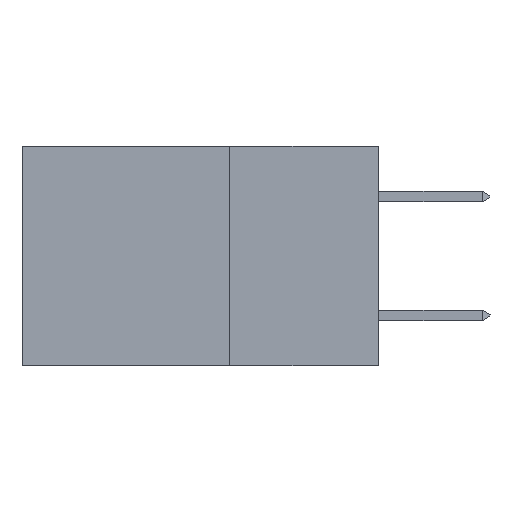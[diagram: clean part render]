
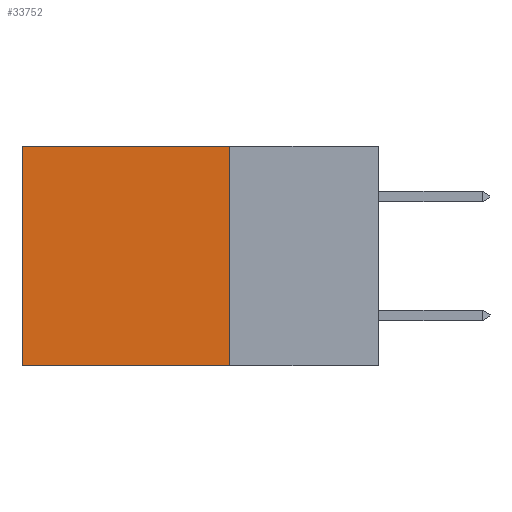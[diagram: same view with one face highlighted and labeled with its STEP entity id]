
A CAD part, left-side view. The second image highlights one B-rep face of the part: STEP entity #33752.
In plain terms, the highlighted planar face has unit normal (-1, 0, 0).
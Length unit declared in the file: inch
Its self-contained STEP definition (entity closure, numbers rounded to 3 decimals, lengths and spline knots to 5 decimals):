
#383 = LINE ( 'NONE', #13626, #21250 ) ;
#1991 = LINE ( 'NONE', #14796, #5744 ) ;
#3336 = VERTEX_POINT ( 'NONE', #23021 ) ;
#4294 = ORIENTED_EDGE ( 'NONE', *, *, #11219, .T. ) ;
#4408 = CARTESIAN_POINT ( 'NONE',  ( 0.298, 0.25, 0. ) ) ;
#4833 = FACE_OUTER_BOUND ( 'NONE', #34404, .T. ) ;
#5744 = VECTOR ( 'NONE', #24946, 39.37008 ) ;
#5864 = EDGE_CURVE ( 'NONE', #24823, #3336, #1991, .T. ) ;
#5874 = CARTESIAN_POINT ( 'NONE',  ( 0.298, 0.25, -0.37 ) ) ;
#6269 = LINE ( 'NONE', #25279, #28749 ) ;
#8579 = LINE ( 'NONE', #21059, #11482 ) ;
#10102 = DIRECTION ( 'NONE',  ( 1., 0., 0. ) ) ;
#10293 = VERTEX_POINT ( 'NONE', #10602 ) ;
#10329 = DIRECTION ( 'NONE',  ( 0., 0., -1. ) ) ;
#10602 = CARTESIAN_POINT ( 'NONE',  ( 0.298, 0.6, 0. ) ) ;
#11219 = EDGE_CURVE ( 'NONE', #10293, #3336, #8579, .T. ) ;
#11482 = VECTOR ( 'NONE', #34122, 39.37008 ) ;
#13626 = CARTESIAN_POINT ( 'NONE',  ( 0.298, 0.25, 0. ) ) ;
#14796 = CARTESIAN_POINT ( 'NONE',  ( 0.298, 0.25, -0.37 ) ) ;
#16840 = EDGE_CURVE ( 'NONE', #27444, #24823, #383, .T. ) ;
#17937 = DIRECTION ( 'NONE',  ( 0., 1., 0. ) ) ;
#20453 = ORIENTED_EDGE ( 'NONE', *, *, #5864, .F. ) ;
#21059 = CARTESIAN_POINT ( 'NONE',  ( 0.298, 0.6, 0. ) ) ;
#21250 = VECTOR ( 'NONE', #24350, 39.37008 ) ;
#23021 = CARTESIAN_POINT ( 'NONE',  ( 0.298, 0.6, -0.37 ) ) ;
#23742 = CARTESIAN_POINT ( 'NONE',  ( 0.298, 0.25, 0. ) ) ;
#24141 = EDGE_CURVE ( 'NONE', #27444, #10293, #6269, .T. ) ;
#24350 = DIRECTION ( 'NONE',  ( 0., 0., -1. ) ) ;
#24823 = VERTEX_POINT ( 'NONE', #5874 ) ;
#24946 = DIRECTION ( 'NONE',  ( 0., 1., 0. ) ) ;
#25074 = ORIENTED_EDGE ( 'NONE', *, *, #24141, .T. ) ;
#25279 = CARTESIAN_POINT ( 'NONE',  ( 0.298, 0.25, 0. ) ) ;
#27444 = VERTEX_POINT ( 'NONE', #4408 ) ;
#28749 = VECTOR ( 'NONE', #17937, 39.37008 ) ;
#29601 = AXIS2_PLACEMENT_3D ( 'NONE', #23742, #10102, #10329 ) ;
#29910 = ORIENTED_EDGE ( 'NONE', *, *, #16840, .F. ) ;
#31677 = PLANE ( 'NONE',  #29601 ) ;
#33752 = ADVANCED_FACE ( 'NONE', ( #4833 ), #31677, .F. ) ;
#34122 = DIRECTION ( 'NONE',  ( 0., 0., -1. ) ) ;
#34404 = EDGE_LOOP ( 'NONE', ( #4294, #20453, #29910, #25074 ) ) ;
